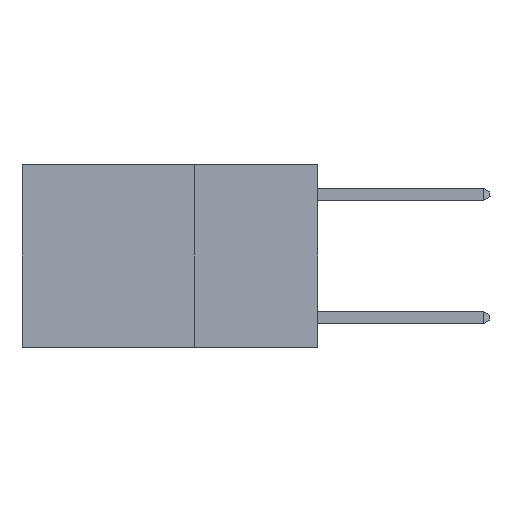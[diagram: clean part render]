
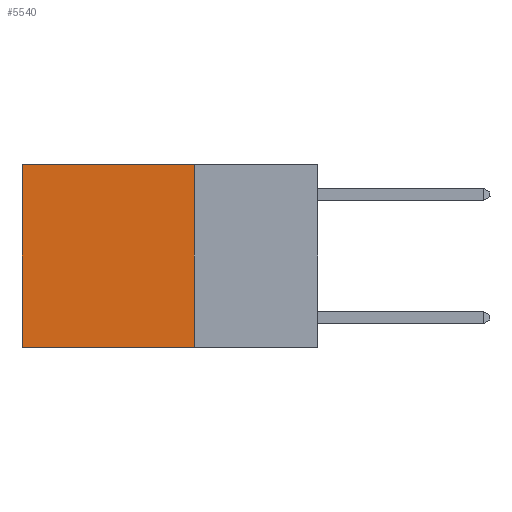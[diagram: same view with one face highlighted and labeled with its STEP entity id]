
A CAD part, left-side view. The second image highlights one B-rep face of the part: STEP entity #5540.
In plain terms, the highlighted planar face has unit normal (-1, 0, 0).
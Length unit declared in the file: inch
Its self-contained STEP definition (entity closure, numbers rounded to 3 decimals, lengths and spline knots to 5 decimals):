
#393 = LINE ( 'NONE', #8874, #10756 ) ;
#933 = EDGE_CURVE ( 'NONE', #10518, #2284, #10383, .T. ) ;
#1038 = EDGE_LOOP ( 'NONE', ( #2966, #6713, #4520, #5456 ) ) ;
#1173 = CARTESIAN_POINT ( 'NONE',  ( 0.2625, 0.6, -0.37 ) ) ;
#1238 = VECTOR ( 'NONE', #9351, 39.37008 ) ;
#1732 = CARTESIAN_POINT ( 'NONE',  ( 0.2625, 0.25, -0.37 ) ) ;
#2284 = VERTEX_POINT ( 'NONE', #1173 ) ;
#2539 = CARTESIAN_POINT ( 'NONE',  ( 0.2625, 0.25, 0. ) ) ;
#2844 = DIRECTION ( 'NONE',  ( 1., 0., 0. ) ) ;
#2917 = VERTEX_POINT ( 'NONE', #3909 ) ;
#2966 = ORIENTED_EDGE ( 'NONE', *, *, #10861, .T. ) ;
#3553 = VERTEX_POINT ( 'NONE', #7937 ) ;
#3909 = CARTESIAN_POINT ( 'NONE',  ( 0.2625, 0.6, 0. ) ) ;
#4195 = DIRECTION ( 'NONE',  ( 0., 1., 0. ) ) ;
#4352 = CARTESIAN_POINT ( 'NONE',  ( 0.2625, 0.25, 0. ) ) ;
#4520 = ORIENTED_EDGE ( 'NONE', *, *, #7398, .F. ) ;
#4730 = DIRECTION ( 'NONE',  ( 0., 0., -1. ) ) ;
#5456 = ORIENTED_EDGE ( 'NONE', *, *, #7485, .T. ) ;
#5457 = CARTESIAN_POINT ( 'NONE',  ( 0.2625, 0.25, 0. ) ) ;
#5540 = ADVANCED_FACE ( 'NONE', ( #7830 ), #7941, .F. ) ;
#5618 = LINE ( 'NONE', #4352, #1238 ) ;
#6713 = ORIENTED_EDGE ( 'NONE', *, *, #933, .F. ) ;
#7398 = EDGE_CURVE ( 'NONE', #3553, #10518, #10374, .T. ) ;
#7485 = EDGE_CURVE ( 'NONE', #3553, #2917, #5618, .T. ) ;
#7830 = FACE_OUTER_BOUND ( 'NONE', #1038, .T. ) ;
#7937 = CARTESIAN_POINT ( 'NONE',  ( 0.2625, 0.25, 0. ) ) ;
#7941 = PLANE ( 'NONE',  #10792 ) ;
#7953 = CARTESIAN_POINT ( 'NONE',  ( 0.2625, 0.25, -0.37 ) ) ;
#8314 = VECTOR ( 'NONE', #10755, 39.37008 ) ;
#8324 = VECTOR ( 'NONE', #4195, 39.37008 ) ;
#8770 = DIRECTION ( 'NONE',  ( 0., 0., -1. ) ) ;
#8874 = CARTESIAN_POINT ( 'NONE',  ( 0.2625, 0.6, 0. ) ) ;
#9351 = DIRECTION ( 'NONE',  ( 0., 1., 0. ) ) ;
#10374 = LINE ( 'NONE', #2539, #8314 ) ;
#10383 = LINE ( 'NONE', #7953, #8324 ) ;
#10518 = VERTEX_POINT ( 'NONE', #1732 ) ;
#10755 = DIRECTION ( 'NONE',  ( 0., 0., -1. ) ) ;
#10756 = VECTOR ( 'NONE', #4730, 39.37008 ) ;
#10792 = AXIS2_PLACEMENT_3D ( 'NONE', #5457, #2844, #8770 ) ;
#10861 = EDGE_CURVE ( 'NONE', #2917, #2284, #393, .T. ) ;
